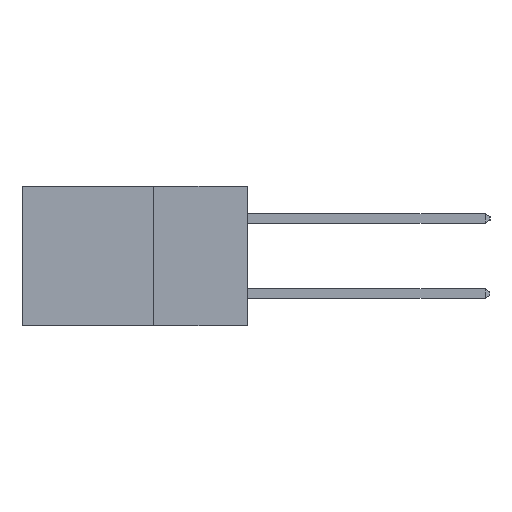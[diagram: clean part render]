
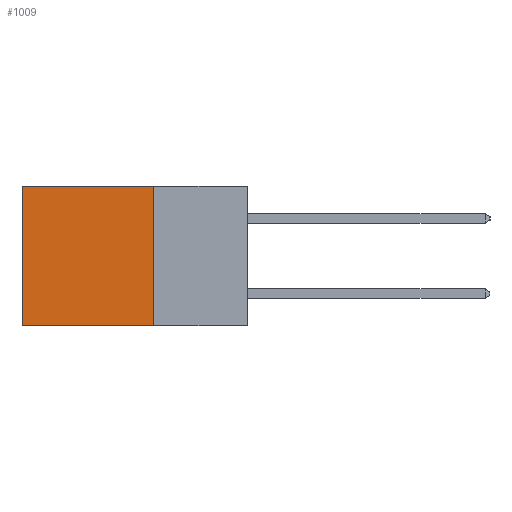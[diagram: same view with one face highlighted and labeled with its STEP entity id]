
A CAD part, left-side view. The second image highlights one B-rep face of the part: STEP entity #1009.
In plain terms, the highlighted planar face has unit normal (-1, 0, 0).
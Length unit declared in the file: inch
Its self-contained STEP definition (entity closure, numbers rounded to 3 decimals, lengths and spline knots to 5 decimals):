
#1009 = ADVANCED_FACE ( 'NONE', ( #9184 ), #3137, .F. ) ;
#1354 = DIRECTION ( 'NONE',  ( 0., 1., 0. ) ) ;
#1731 = EDGE_CURVE ( 'NONE', #11393, #12822, #2840, .T. ) ;
#1837 = CARTESIAN_POINT ( 'NONE',  ( 0.298, 0.6, -0.37 ) ) ;
#1934 = LINE ( 'NONE', #6517, #7281 ) ;
#2086 = DIRECTION ( 'NONE',  ( 1., 0., 0. ) ) ;
#2203 = LINE ( 'NONE', #5202, #7570 ) ;
#2658 = CARTESIAN_POINT ( 'NONE',  ( 0.298, 0.25, 0. ) ) ;
#2840 = LINE ( 'NONE', #3908, #11010 ) ;
#3137 = PLANE ( 'NONE',  #11749 ) ;
#3307 = CARTESIAN_POINT ( 'NONE',  ( 0.298, 0.25, -0.37 ) ) ;
#3744 = VERTEX_POINT ( 'NONE', #7373 ) ;
#3908 = CARTESIAN_POINT ( 'NONE',  ( 0.298, 0.6, 0. ) ) ;
#3964 = LINE ( 'NONE', #8817, #6525 ) ;
#4539 = EDGE_CURVE ( 'NONE', #3744, #13046, #1934, .T. ) ;
#5004 = EDGE_LOOP ( 'NONE', ( #5044, #5259, #6397, #6591 ) ) ;
#5044 = ORIENTED_EDGE ( 'NONE', *, *, #1731, .T. ) ;
#5202 = CARTESIAN_POINT ( 'NONE',  ( 0.298, 0.25, -0.37 ) ) ;
#5259 = ORIENTED_EDGE ( 'NONE', *, *, #6772, .F. ) ;
#5795 = DIRECTION ( 'NONE',  ( 0., 0., -1. ) ) ;
#6331 = DIRECTION ( 'NONE',  ( 0., 0., -1. ) ) ;
#6397 = ORIENTED_EDGE ( 'NONE', *, *, #4539, .F. ) ;
#6517 = CARTESIAN_POINT ( 'NONE',  ( 0.298, 0.25, 0. ) ) ;
#6525 = VECTOR ( 'NONE', #1354, 39.37008 ) ;
#6591 = ORIENTED_EDGE ( 'NONE', *, *, #9399, .T. ) ;
#6772 = EDGE_CURVE ( 'NONE', #13046, #12822, #2203, .T. ) ;
#7281 = VECTOR ( 'NONE', #10735, 39.37008 ) ;
#7373 = CARTESIAN_POINT ( 'NONE',  ( 0.298, 0.25, 0. ) ) ;
#7570 = VECTOR ( 'NONE', #13720, 39.37008 ) ;
#8764 = CARTESIAN_POINT ( 'NONE',  ( 0.298, 0.6, 0. ) ) ;
#8817 = CARTESIAN_POINT ( 'NONE',  ( 0.298, 0.25, 0. ) ) ;
#9184 = FACE_OUTER_BOUND ( 'NONE', #5004, .T. ) ;
#9399 = EDGE_CURVE ( 'NONE', #3744, #11393, #3964, .T. ) ;
#10735 = DIRECTION ( 'NONE',  ( 0., 0., -1. ) ) ;
#11010 = VECTOR ( 'NONE', #6331, 39.37008 ) ;
#11393 = VERTEX_POINT ( 'NONE', #8764 ) ;
#11749 = AXIS2_PLACEMENT_3D ( 'NONE', #2658, #2086, #5795 ) ;
#12822 = VERTEX_POINT ( 'NONE', #1837 ) ;
#13046 = VERTEX_POINT ( 'NONE', #3307 ) ;
#13720 = DIRECTION ( 'NONE',  ( 0., 1., 0. ) ) ;
